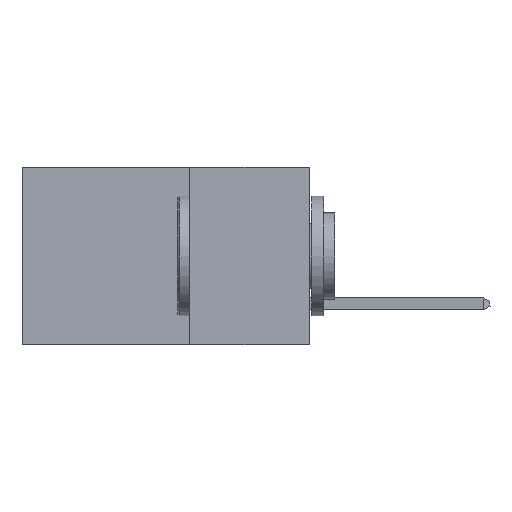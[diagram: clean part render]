
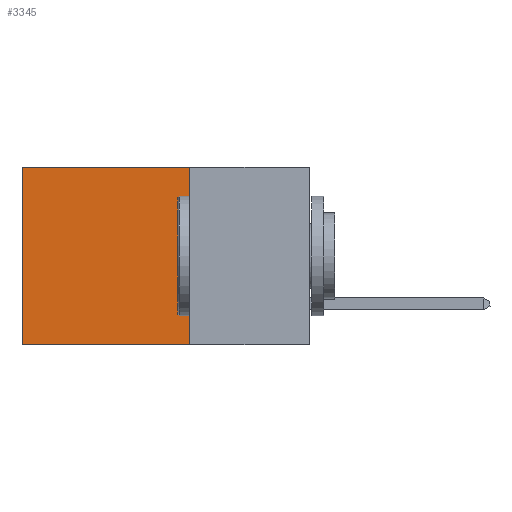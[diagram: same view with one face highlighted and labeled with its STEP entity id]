
A CAD part, left-side view. The second image highlights one B-rep face of the part: STEP entity #3345.
In plain terms, the highlighted planar face has unit normal (-1, 0, 0).
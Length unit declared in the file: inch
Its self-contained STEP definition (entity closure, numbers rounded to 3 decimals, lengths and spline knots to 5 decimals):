
#306 = AXIS2_PLACEMENT_3D ( 'NONE', #7810, #7724, #7722 ) ;
#635 = VECTOR ( 'NONE', #2146, 39.37008 ) ;
#764 = VECTOR ( 'NONE', #1554, 39.37008 ) ;
#1060 = ORIENTED_EDGE ( 'NONE', *, *, #2033, .T. ) ;
#1127 = ORIENTED_EDGE ( 'NONE', *, *, #2753, .F. ) ;
#1187 = ORIENTED_EDGE ( 'NONE', *, *, #6276, .F. ) ;
#1229 = VECTOR ( 'NONE', #3672, 39.37008 ) ;
#1251 = ORIENTED_EDGE ( 'NONE', *, *, #1416, .T. ) ;
#1323 = VERTEX_POINT ( 'NONE', #4970 ) ;
#1416 = EDGE_CURVE ( 'NONE', #1323, #7502, #5488, .T. ) ;
#1554 = DIRECTION ( 'NONE',  ( 0., 1., 0. ) ) ;
#1598 = CARTESIAN_POINT ( 'NONE',  ( 0.2875, 0.6, 0. ) ) ;
#1617 = CARTESIAN_POINT ( 'NONE',  ( 0.2875, 0.25, -0.37 ) ) ;
#1877 = VECTOR ( 'NONE', #2665, 39.37008 ) ;
#2033 = EDGE_CURVE ( 'NONE', #7502, #5777, #2682, .T. ) ;
#2146 = DIRECTION ( 'NONE',  ( 0., 0., -1. ) ) ;
#2159 = CARTESIAN_POINT ( 'NONE',  ( 0.2875, 0.6, 0. ) ) ;
#2429 = CARTESIAN_POINT ( 'NONE',  ( 0.2875, 0.25, 0. ) ) ;
#2665 = DIRECTION ( 'NONE',  ( 0., 0., -1. ) ) ;
#2682 = LINE ( 'NONE', #2159, #635 ) ;
#2753 = EDGE_CURVE ( 'NONE', #4809, #5777, #4852, .T. ) ;
#3345 = ADVANCED_FACE ( 'NONE', ( #5676 ), #7777, .F. ) ;
#3425 = CARTESIAN_POINT ( 'NONE',  ( 0.2875, 0.25, 0. ) ) ;
#3672 = DIRECTION ( 'NONE',  ( 0., 1., 0. ) ) ;
#4809 = VERTEX_POINT ( 'NONE', #9226 ) ;
#4852 = LINE ( 'NONE', #1617, #764 ) ;
#4970 = CARTESIAN_POINT ( 'NONE',  ( 0.2875, 0.25, 0. ) ) ;
#5488 = LINE ( 'NONE', #3425, #1229 ) ;
#5676 = FACE_OUTER_BOUND ( 'NONE', #8169, .T. ) ;
#5777 = VERTEX_POINT ( 'NONE', #8304 ) ;
#6276 = EDGE_CURVE ( 'NONE', #1323, #4809, #6657, .T. ) ;
#6657 = LINE ( 'NONE', #2429, #1877 ) ;
#7502 = VERTEX_POINT ( 'NONE', #1598 ) ;
#7722 = DIRECTION ( 'NONE',  ( 0., 0., -1. ) ) ;
#7724 = DIRECTION ( 'NONE',  ( 1., 0., 0. ) ) ;
#7777 = PLANE ( 'NONE',  #306 ) ;
#7810 = CARTESIAN_POINT ( 'NONE',  ( 0.2875, 0.25, 0. ) ) ;
#8169 = EDGE_LOOP ( 'NONE', ( #1060, #1127, #1187, #1251 ) ) ;
#8304 = CARTESIAN_POINT ( 'NONE',  ( 0.2875, 0.6, -0.37 ) ) ;
#9226 = CARTESIAN_POINT ( 'NONE',  ( 0.2875, 0.25, -0.37 ) ) ;
